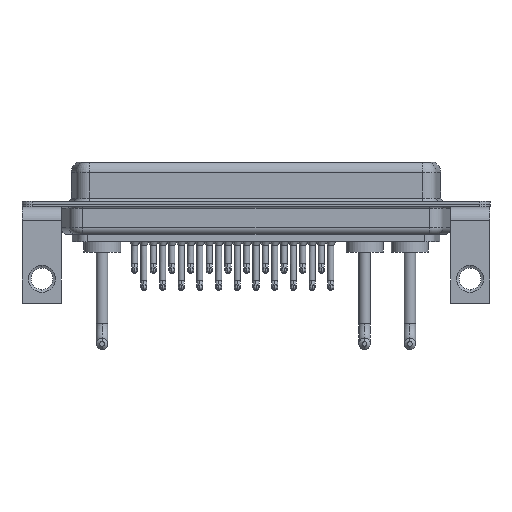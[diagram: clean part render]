
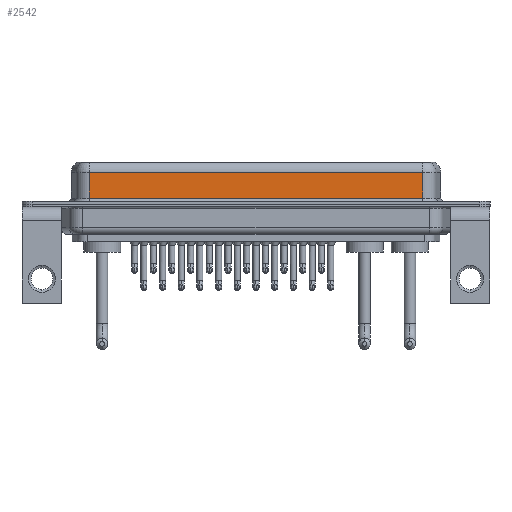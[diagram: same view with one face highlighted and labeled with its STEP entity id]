
A CAD part, front view. The second image highlights one B-rep face of the part: STEP entity #2542.
In plain terms, the highlighted planar face has unit normal (0, -1, 0).
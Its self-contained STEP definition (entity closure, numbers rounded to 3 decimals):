
#555 = CARTESIAN_POINT ( 'NONE',  ( 56.462, -3.95, 0.9 ) ) ;
#1923 = ORIENTED_EDGE ( 'NONE', *, *, #7123, .F. ) ;
#2542 = ADVANCED_FACE ( 'NONE', ( #18466 ), #22454, .F. ) ;
#2649 = CARTESIAN_POINT ( 'NONE',  ( 7.038, -3.95, 4.65 ) ) ;
#3717 = LINE ( 'NONE', #19106, #7518 ) ;
#3923 = LINE ( 'NONE', #19072, #11747 ) ;
#4097 = DIRECTION ( 'NONE',  ( 0., 0., -1. ) ) ;
#7123 = EDGE_CURVE ( 'NONE', #11958, #12592, #13167, .T. ) ;
#7518 = VECTOR ( 'NONE', #13529, 1000. ) ;
#7699 = VECTOR ( 'NONE', #4097, 1000. ) ;
#7850 = AXIS2_PLACEMENT_3D ( 'NONE', #20578, #22215, #21966 ) ;
#8429 = VERTEX_POINT ( 'NONE', #23356 ) ;
#9243 = VECTOR ( 'NONE', #16760, 1000. ) ;
#11459 = EDGE_CURVE ( 'NONE', #8429, #12592, #3717, .T. ) ;
#11747 = VECTOR ( 'NONE', #17228, 1000. ) ;
#11958 = VERTEX_POINT ( 'NONE', #15347 ) ;
#12592 = VERTEX_POINT ( 'NONE', #555 ) ;
#13167 = LINE ( 'NONE', #15645, #7699 ) ;
#13529 = DIRECTION ( 'NONE',  ( 1., 0., 0. ) ) ;
#14996 = LINE ( 'NONE', #22354, #9243 ) ;
#15347 = CARTESIAN_POINT ( 'NONE',  ( 56.462, -3.95, 4.65 ) ) ;
#15645 = CARTESIAN_POINT ( 'NONE',  ( 56.462, -3.95, 6.4 ) ) ;
#16760 = DIRECTION ( 'NONE',  ( -1., 0., 0. ) ) ;
#17228 = DIRECTION ( 'NONE',  ( 0., 0., -1. ) ) ;
#17321 = EDGE_CURVE ( 'NONE', #11958, #22120, #14996, .T. ) ;
#17595 = EDGE_LOOP ( 'NONE', ( #1923, #19234, #17995, #24081 ) ) ;
#17995 = ORIENTED_EDGE ( 'NONE', *, *, #19375, .T. ) ;
#18466 = FACE_OUTER_BOUND ( 'NONE', #17595, .T. ) ;
#19072 = CARTESIAN_POINT ( 'NONE',  ( 7.038, -3.95, 6.4 ) ) ;
#19106 = CARTESIAN_POINT ( 'NONE',  ( 56.462, -3.95, 0.9 ) ) ;
#19234 = ORIENTED_EDGE ( 'NONE', *, *, #17321, .T. ) ;
#19375 = EDGE_CURVE ( 'NONE', #22120, #8429, #3923, .T. ) ;
#20578 = CARTESIAN_POINT ( 'NONE',  ( 56.462, -3.95, 6.4 ) ) ;
#21966 = DIRECTION ( 'NONE',  ( 0., 0., 1. ) ) ;
#22120 = VERTEX_POINT ( 'NONE', #2649 ) ;
#22215 = DIRECTION ( 'NONE',  ( 0., 1., 0. ) ) ;
#22354 = CARTESIAN_POINT ( 'NONE',  ( 56.462, -3.95, 4.65 ) ) ;
#22454 = PLANE ( 'NONE',  #7850 ) ;
#23356 = CARTESIAN_POINT ( 'NONE',  ( 7.038, -3.95, 0.9 ) ) ;
#24081 = ORIENTED_EDGE ( 'NONE', *, *, #11459, .T. ) ;
